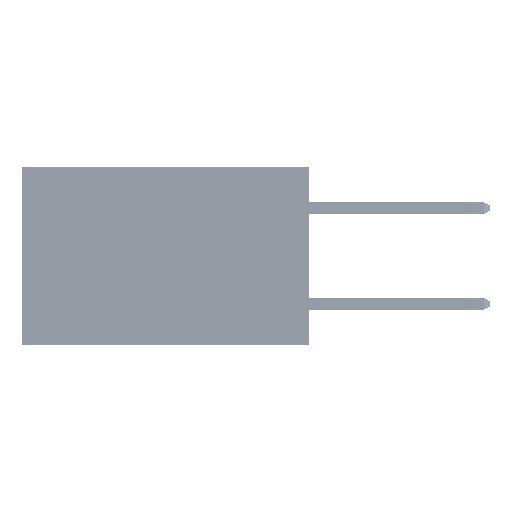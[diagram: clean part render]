
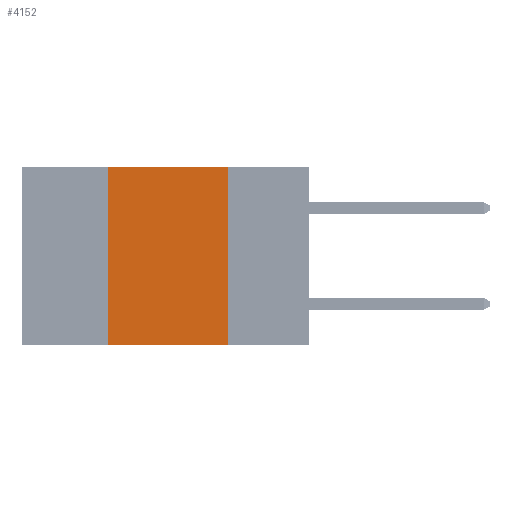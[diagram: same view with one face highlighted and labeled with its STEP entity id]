
A CAD part, left-side view. The second image highlights one B-rep face of the part: STEP entity #4152.
In plain terms, the highlighted planar face has unit normal (-1, 0, 0).
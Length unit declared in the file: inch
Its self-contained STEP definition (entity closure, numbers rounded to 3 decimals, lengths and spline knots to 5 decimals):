
#1211 = DIRECTION ( 'NONE',  ( 0., 0., -1. ) ) ;
#1862 = LINE ( 'NONE', #41288, #47559 ) ;
#3415 = CARTESIAN_POINT ( 'NONE',  ( 0., 0.6, 0. ) ) ;
#3467 = EDGE_CURVE ( 'NONE', #23119, #46545, #1862, .T. ) ;
#4152 = ADVANCED_FACE ( 'NONE', ( #11946 ), #12178, .F. ) ;
#8633 = EDGE_CURVE ( 'NONE', #23119, #25225, #20415, .T. ) ;
#10301 = CARTESIAN_POINT ( 'NONE',  ( 0., 0.17, -0.37 ) ) ;
#10552 = VECTOR ( 'NONE', #1211, 39.37008 ) ;
#11946 = FACE_OUTER_BOUND ( 'NONE', #20237, .T. ) ;
#12178 = PLANE ( 'NONE',  #39210 ) ;
#13616 = CARTESIAN_POINT ( 'NONE',  ( 0., 0.17, 0. ) ) ;
#16213 = LINE ( 'NONE', #13616, #10552 ) ;
#16239 = CARTESIAN_POINT ( 'NONE',  ( 0., 0.6, 0. ) ) ;
#16371 = DIRECTION ( 'NONE',  ( 0., 0., 1. ) ) ;
#17072 = CARTESIAN_POINT ( 'NONE',  ( 0., 0.42, 0. ) ) ;
#18714 = VERTEX_POINT ( 'NONE', #46059 ) ;
#20237 = EDGE_LOOP ( 'NONE', ( #39172, #24110, #34050, #37160 ) ) ;
#20365 = DIRECTION ( 'NONE',  ( 1., 0., 0. ) ) ;
#20415 = LINE ( 'NONE', #17072, #44503 ) ;
#23119 = VERTEX_POINT ( 'NONE', #45035 ) ;
#24110 = ORIENTED_EDGE ( 'NONE', *, *, #44168, .F. ) ;
#24440 = DIRECTION ( 'NONE',  ( 0., 0., -1. ) ) ;
#25225 = VERTEX_POINT ( 'NONE', #31004 ) ;
#31004 = CARTESIAN_POINT ( 'NONE',  ( 0., 0.42, 0. ) ) ;
#33178 = LINE ( 'NONE', #3415, #43330 ) ;
#34050 = ORIENTED_EDGE ( 'NONE', *, *, #8633, .F. ) ;
#36715 = DIRECTION ( 'NONE',  ( 0., -1., 0. ) ) ;
#37160 = ORIENTED_EDGE ( 'NONE', *, *, #3467, .T. ) ;
#39172 = ORIENTED_EDGE ( 'NONE', *, *, #48245, .F. ) ;
#39210 = AXIS2_PLACEMENT_3D ( 'NONE', #16239, #20365, #24440 ) ;
#41288 = CARTESIAN_POINT ( 'NONE',  ( 0., 0.6, -0.37 ) ) ;
#43330 = VECTOR ( 'NONE', #52172, 39.37008 ) ;
#44168 = EDGE_CURVE ( 'NONE', #25225, #18714, #33178, .T. ) ;
#44503 = VECTOR ( 'NONE', #16371, 39.37008 ) ;
#45035 = CARTESIAN_POINT ( 'NONE',  ( 0., 0.42, -0.37 ) ) ;
#46059 = CARTESIAN_POINT ( 'NONE',  ( 0., 0.17, 0. ) ) ;
#46545 = VERTEX_POINT ( 'NONE', #10301 ) ;
#47559 = VECTOR ( 'NONE', #36715, 39.37008 ) ;
#48245 = EDGE_CURVE ( 'NONE', #18714, #46545, #16213, .T. ) ;
#52172 = DIRECTION ( 'NONE',  ( 0., -1., 0. ) ) ;
